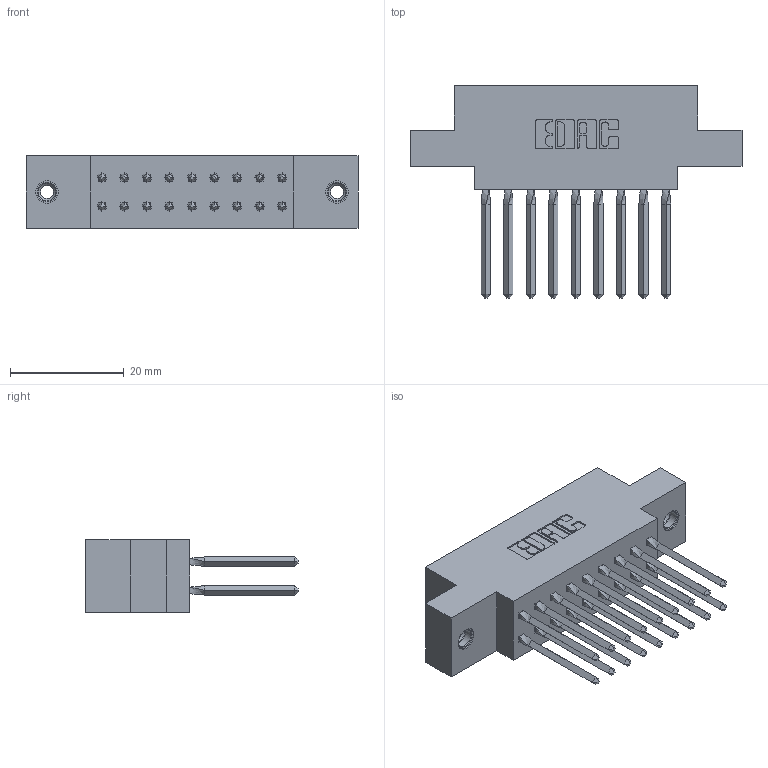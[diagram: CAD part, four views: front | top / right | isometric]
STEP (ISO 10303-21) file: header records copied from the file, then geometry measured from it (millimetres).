
FILE_DESCRIPTION (( 'STEP AP203' ), '1' );
FILE_NAME ('317-018-540-878.STEP', '2020-02-27T16:03:28', ( '' ), ( '' ), 'SwSTEP 2.0', 'SolidWorks 2016', '' );
FILE_SCHEMA (( 'CONFIG_CONTROL_DESIGN' ));
Length unit declared in the file: inch
Products named in the file (4): 345-250-001_345-250-003-102; 317-018-540-878; 317-290-001_540; 317 Part_.156 Dia - TI
Assembly tree (21 placements, depth 2):
  317-018-540-878
    317 Part_.156 Dia - TI
    317-290-001_540  x18
    345-250-001_345-250-003-102  x2
Bounding box: 58.37 x 37.34 x 12.7 mm (x, y, z)
Volume: 8673.9 mm3; surface area: 11707.7 mm2
Topology: 21 solids, 21 shells, 1764 faces, 4857 edges, 3128 vertices
Faces by surface type: plane 1404, cylinder 272, bspline 72, cone 12, torus 4
Entity records: 18799 total; most frequent: CARTESIAN_POINT 3662, ORIENTED_EDGE 3154, DIRECTION 2677, EDGE_CURVE 1577, VECTOR 1301, LINE 1301, VERTEX_POINT 1041, AXIS2_PLACEMENT_3D 688
